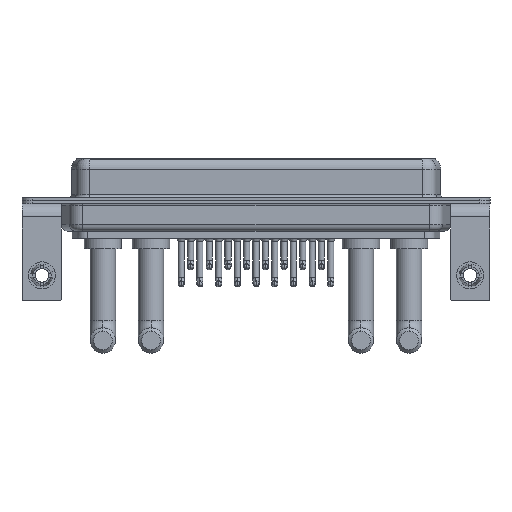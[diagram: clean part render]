
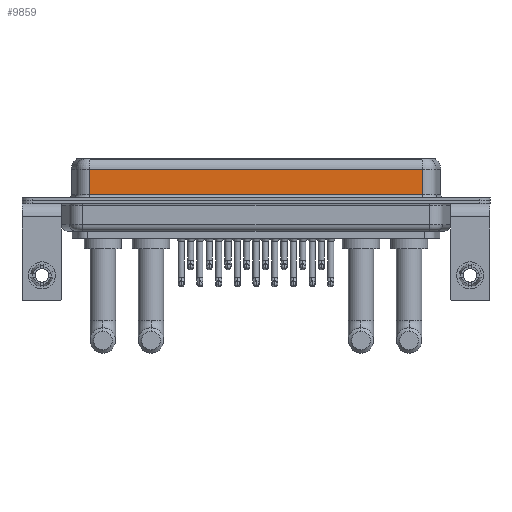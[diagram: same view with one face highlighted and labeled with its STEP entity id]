
A CAD part, front view. The second image highlights one B-rep face of the part: STEP entity #9859.
In plain terms, the highlighted planar face has unit normal (0, -1, 0).
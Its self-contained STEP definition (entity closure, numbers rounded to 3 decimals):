
#152 = FACE_OUTER_BOUND ( 'NONE', #20434, .T. ) ;
#970 = VECTOR ( 'NONE', #17433, 1000. ) ;
#1042 = VERTEX_POINT ( 'NONE', #6176 ) ;
#1571 = DIRECTION ( 'NONE',  ( 1., 0., 0. ) ) ;
#1608 = ORIENTED_EDGE ( 'NONE', *, *, #13119, .F. ) ;
#1897 = ORIENTED_EDGE ( 'NONE', *, *, #2915, .T. ) ;
#2030 = VERTEX_POINT ( 'NONE', #13530 ) ;
#2364 = DIRECTION ( 'NONE',  ( 0., 0., -1. ) ) ;
#2915 = EDGE_CURVE ( 'NONE', #1042, #4475, #13805, .T. ) ;
#3734 = DIRECTION ( 'NONE',  ( 0., 1., 0. ) ) ;
#4475 = VERTEX_POINT ( 'NONE', #21537 ) ;
#5284 = VECTOR ( 'NONE', #2364, 1000. ) ;
#5950 = CARTESIAN_POINT ( 'NONE',  ( 7.038, -3.95, 6.4 ) ) ;
#6176 = CARTESIAN_POINT ( 'NONE',  ( 56.462, -3.95, 4.65 ) ) ;
#7570 = CARTESIAN_POINT ( 'NONE',  ( 56.462, -3.95, 6.4 ) ) ;
#7687 = PLANE ( 'NONE',  #23333 ) ;
#9112 = LINE ( 'NONE', #18234, #16045 ) ;
#9673 = CARTESIAN_POINT ( 'NONE',  ( 56.462, -3.95, 6.4 ) ) ;
#9859 = ADVANCED_FACE ( 'NONE', ( #152 ), #7687, .F. ) ;
#11651 = LINE ( 'NONE', #9673, #970 ) ;
#11972 = DIRECTION ( 'NONE',  ( -1., 0., 0. ) ) ;
#13119 = EDGE_CURVE ( 'NONE', #1042, #18035, #11651, .T. ) ;
#13530 = CARTESIAN_POINT ( 'NONE',  ( 7.038, -3.95, 0.9 ) ) ;
#13805 = LINE ( 'NONE', #15793, #21702 ) ;
#14920 = CARTESIAN_POINT ( 'NONE',  ( 56.462, -3.95, 0.9 ) ) ;
#15793 = CARTESIAN_POINT ( 'NONE',  ( 56.462, -3.95, 4.65 ) ) ;
#16045 = VECTOR ( 'NONE', #1571, 1000. ) ;
#16137 = EDGE_CURVE ( 'NONE', #4475, #2030, #22847, .T. ) ;
#17433 = DIRECTION ( 'NONE',  ( 0., 0., -1. ) ) ;
#18035 = VERTEX_POINT ( 'NONE', #14920 ) ;
#18234 = CARTESIAN_POINT ( 'NONE',  ( 56.462, -3.95, 0.9 ) ) ;
#18487 = EDGE_CURVE ( 'NONE', #2030, #18035, #9112, .T. ) ;
#19031 = DIRECTION ( 'NONE',  ( 0., 0., 1. ) ) ;
#19394 = ORIENTED_EDGE ( 'NONE', *, *, #16137, .T. ) ;
#20434 = EDGE_LOOP ( 'NONE', ( #1608, #1897, #19394, #22734 ) ) ;
#21537 = CARTESIAN_POINT ( 'NONE',  ( 7.038, -3.95, 4.65 ) ) ;
#21702 = VECTOR ( 'NONE', #11972, 1000. ) ;
#22734 = ORIENTED_EDGE ( 'NONE', *, *, #18487, .T. ) ;
#22847 = LINE ( 'NONE', #5950, #5284 ) ;
#23333 = AXIS2_PLACEMENT_3D ( 'NONE', #7570, #3734, #19031 ) ;
